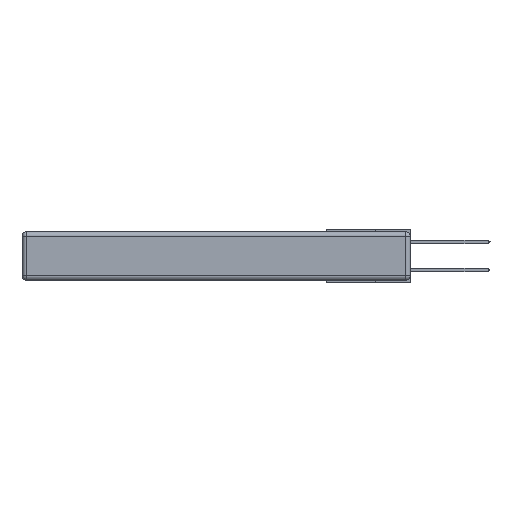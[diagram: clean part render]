
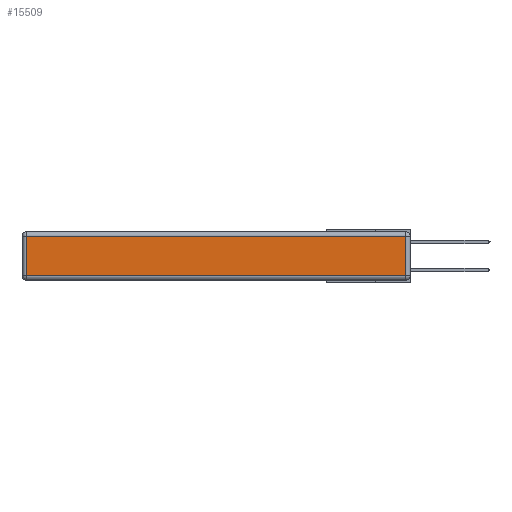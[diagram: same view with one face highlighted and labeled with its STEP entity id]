
A CAD part, left-side view. The second image highlights one B-rep face of the part: STEP entity #15509.
In plain terms, the highlighted planar face has unit normal (-1, 0, 0).
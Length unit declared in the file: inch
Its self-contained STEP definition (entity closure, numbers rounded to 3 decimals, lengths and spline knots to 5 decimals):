
#346 = PLANE ( 'NONE',  #12222 ) ;
#672 = ORIENTED_EDGE ( 'NONE', *, *, #4997, .T. ) ;
#990 = VERTEX_POINT ( 'NONE', #22284 ) ;
#1427 = ORIENTED_EDGE ( 'NONE', *, *, #9478, .T. ) ;
#2035 = EDGE_CURVE ( 'NONE', #990, #9650, #11384, .T. ) ;
#2113 = CARTESIAN_POINT ( 'NONE',  ( 0., 0., -0.343 ) ) ;
#3853 = VECTOR ( 'NONE', #9027, 39.37008 ) ;
#3961 = CARTESIAN_POINT ( 'NONE',  ( 0., 0., -0.313 ) ) ;
#4328 = FACE_OUTER_BOUND ( 'NONE', #13902, .T. ) ;
#4997 = EDGE_CURVE ( 'NONE', #9650, #13406, #18608, .T. ) ;
#6200 = CARTESIAN_POINT ( 'NONE',  ( 0., 2.72, -0.313 ) ) ;
#6954 = CARTESIAN_POINT ( 'NONE',  ( 0., 0.03, -0.03 ) ) ;
#6989 = CARTESIAN_POINT ( 'NONE',  ( 0., 0.03, -0.343 ) ) ;
#7630 = DIRECTION ( 'NONE',  ( 0., -1., 0. ) ) ;
#9027 = DIRECTION ( 'NONE',  ( 0., 0., 1. ) ) ;
#9478 = EDGE_CURVE ( 'NONE', #13406, #20060, #15593, .T. ) ;
#9650 = VERTEX_POINT ( 'NONE', #6200 ) ;
#9690 = CARTESIAN_POINT ( 'NONE',  ( 0., 2.72, -0.343 ) ) ;
#9958 = CARTESIAN_POINT ( 'NONE',  ( 0., 2.75, -0.03 ) ) ;
#10163 = EDGE_CURVE ( 'NONE', #20060, #990, #20173, .T. ) ;
#11384 = LINE ( 'NONE', #9690, #18607 ) ;
#12222 = AXIS2_PLACEMENT_3D ( 'NONE', #2113, #14628, #17886 ) ;
#13311 = VECTOR ( 'NONE', #7630, 39.37008 ) ;
#13406 = VERTEX_POINT ( 'NONE', #15607 ) ;
#13902 = EDGE_LOOP ( 'NONE', ( #672, #1427, #16776, #18450 ) ) ;
#14628 = DIRECTION ( 'NONE',  ( -1., 0., 0. ) ) ;
#15098 = DIRECTION ( 'NONE',  ( 0., 0., -1. ) ) ;
#15509 = ADVANCED_FACE ( 'NONE', ( #4328 ), #346, .T. ) ;
#15593 = LINE ( 'NONE', #6989, #3853 ) ;
#15607 = CARTESIAN_POINT ( 'NONE',  ( 0., 0.03, -0.313 ) ) ;
#16776 = ORIENTED_EDGE ( 'NONE', *, *, #10163, .T. ) ;
#17886 = DIRECTION ( 'NONE',  ( 0., 0., 1. ) ) ;
#18450 = ORIENTED_EDGE ( 'NONE', *, *, #2035, .T. ) ;
#18607 = VECTOR ( 'NONE', #15098, 39.37008 ) ;
#18608 = LINE ( 'NONE', #3961, #13311 ) ;
#20060 = VERTEX_POINT ( 'NONE', #6954 ) ;
#20173 = LINE ( 'NONE', #9958, #21009 ) ;
#20686 = DIRECTION ( 'NONE',  ( 0., 1., 0. ) ) ;
#21009 = VECTOR ( 'NONE', #20686, 39.37008 ) ;
#22284 = CARTESIAN_POINT ( 'NONE',  ( 0., 2.72, -0.03 ) ) ;
